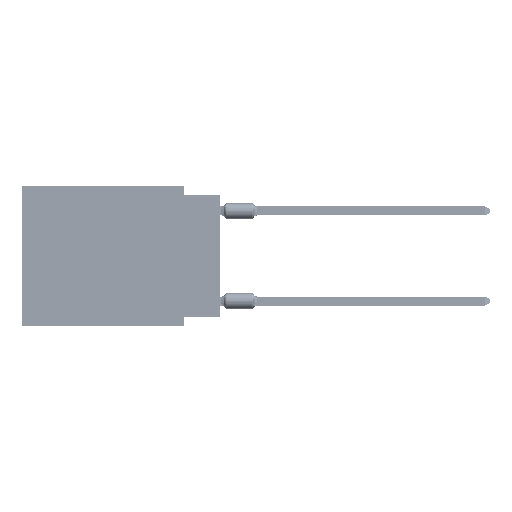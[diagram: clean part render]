
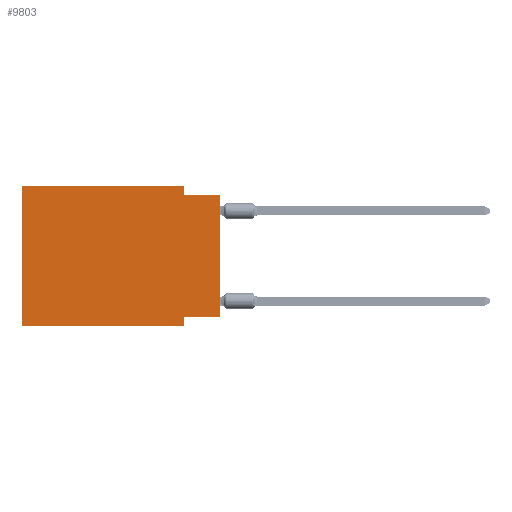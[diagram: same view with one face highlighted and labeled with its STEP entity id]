
A CAD part, left-side view. The second image highlights one B-rep face of the part: STEP entity #9803.
In plain terms, the highlighted planar face has unit normal (-1, 0, 0).
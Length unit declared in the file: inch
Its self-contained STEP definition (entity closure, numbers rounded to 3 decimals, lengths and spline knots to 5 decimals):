
#2476 = CARTESIAN_POINT ( 'NONE',  ( 0., 0.55, 0. ) ) ;
#2557 = ORIENTED_EDGE ( 'NONE', *, *, #18526, .F. ) ;
#5214 = VECTOR ( 'NONE', #5764, 39.37008 ) ;
#5764 = DIRECTION ( 'NONE',  ( 0., 0., 1. ) ) ;
#6551 = EDGE_CURVE ( 'NONE', #72906, #56817, #44185, .T. ) ;
#7378 = AXIS2_PLACEMENT_3D ( 'NONE', #44216, #70729, #11184 ) ;
#8874 = DIRECTION ( 'NONE',  ( 0., 1., 0. ) ) ;
#9182 = VERTEX_POINT ( 'NONE', #49129 ) ;
#9803 = ADVANCED_FACE ( 'NONE', ( #65923 ), #12458, .F. ) ;
#10579 = VECTOR ( 'NONE', #21140, 39.37008 ) ;
#11184 = DIRECTION ( 'NONE',  ( 0., 0., -1. ) ) ;
#11274 = DIRECTION ( 'NONE',  ( 0., 0., -1. ) ) ;
#12458 = PLANE ( 'NONE',  #7378 ) ;
#12565 = ORIENTED_EDGE ( 'NONE', *, *, #36062, .F. ) ;
#16744 = LINE ( 'NONE', #42427, #64588 ) ;
#16815 = CARTESIAN_POINT ( 'NONE',  ( 0., 0.55, -0.39 ) ) ;
#18526 = EDGE_CURVE ( 'NONE', #60700, #67785, #37793, .T. ) ;
#18814 = CARTESIAN_POINT ( 'NONE',  ( 0., 0., 0. ) ) ;
#21140 = DIRECTION ( 'NONE',  ( 0., -1., 0. ) ) ;
#21611 = DIRECTION ( 'NONE',  ( 0., 0., 1. ) ) ;
#21660 = EDGE_CURVE ( 'NONE', #38051, #60700, #54175, .T. ) ;
#21987 = CARTESIAN_POINT ( 'NONE',  ( 0., 0., -0.025 ) ) ;
#22419 = DIRECTION ( 'NONE',  ( 0., 0., -1. ) ) ;
#23654 = VERTEX_POINT ( 'NONE', #81023 ) ;
#24294 = VECTOR ( 'NONE', #11274, 39.37008 ) ;
#35028 = ORIENTED_EDGE ( 'NONE', *, *, #42884, .F. ) ;
#35190 = VECTOR ( 'NONE', #60655, 39.37008 ) ;
#36062 = EDGE_CURVE ( 'NONE', #67785, #23654, #40664, .T. ) ;
#36377 = DIRECTION ( 'NONE',  ( 0., -1., 0. ) ) ;
#36753 = VECTOR ( 'NONE', #36377, 39.37008 ) ;
#37793 = LINE ( 'NONE', #82538, #24294 ) ;
#38051 = VERTEX_POINT ( 'NONE', #59621 ) ;
#40232 = CARTESIAN_POINT ( 'NONE',  ( 0., 0.1, -0.39 ) ) ;
#40664 = LINE ( 'NONE', #21987, #35190 ) ;
#41087 = EDGE_LOOP ( 'NONE', ( #51823, #12565, #2557, #74604, #63601, #71920, #53880, #35028 ) ) ;
#42427 = CARTESIAN_POINT ( 'NONE',  ( 0., 0.1, -0.39 ) ) ;
#42884 = EDGE_CURVE ( 'NONE', #85703, #9182, #54952, .T. ) ;
#43072 = EDGE_CURVE ( 'NONE', #85703, #23654, #64460, .T. ) ;
#44185 = LINE ( 'NONE', #16815, #36753 ) ;
#44216 = CARTESIAN_POINT ( 'NONE',  ( 0., 0.55, 0. ) ) ;
#48211 = CARTESIAN_POINT ( 'NONE',  ( 0., 0.1, -0.025 ) ) ;
#49129 = CARTESIAN_POINT ( 'NONE',  ( 0., 0.1, -0.365 ) ) ;
#49330 = CARTESIAN_POINT ( 'NONE',  ( 0., 0.55, -0.39 ) ) ;
#49957 = CARTESIAN_POINT ( 'NONE',  ( 0., 0.1, 0. ) ) ;
#51823 = ORIENTED_EDGE ( 'NONE', *, *, #43072, .T. ) ;
#52406 = VECTOR ( 'NONE', #8874, 39.37008 ) ;
#53577 = EDGE_CURVE ( 'NONE', #9182, #56817, #16744, .T. ) ;
#53880 = ORIENTED_EDGE ( 'NONE', *, *, #53577, .F. ) ;
#54175 = LINE ( 'NONE', #75010, #10579 ) ;
#54952 = LINE ( 'NONE', #81416, #52406 ) ;
#56530 = CARTESIAN_POINT ( 'NONE',  ( 0., 0., -0.365 ) ) ;
#56817 = VERTEX_POINT ( 'NONE', #40232 ) ;
#59621 = CARTESIAN_POINT ( 'NONE',  ( 0., 0.55, 0. ) ) ;
#60655 = DIRECTION ( 'NONE',  ( 0., -1., 0. ) ) ;
#60700 = VERTEX_POINT ( 'NONE', #49957 ) ;
#62084 = EDGE_CURVE ( 'NONE', #72906, #38051, #81098, .T. ) ;
#63601 = ORIENTED_EDGE ( 'NONE', *, *, #62084, .F. ) ;
#64460 = LINE ( 'NONE', #18814, #5214 ) ;
#64588 = VECTOR ( 'NONE', #22419, 39.37008 ) ;
#65923 = FACE_OUTER_BOUND ( 'NONE', #41087, .T. ) ;
#67785 = VERTEX_POINT ( 'NONE', #48211 ) ;
#70729 = DIRECTION ( 'NONE',  ( 1., 0., 0. ) ) ;
#71920 = ORIENTED_EDGE ( 'NONE', *, *, #6551, .T. ) ;
#72906 = VERTEX_POINT ( 'NONE', #49330 ) ;
#74604 = ORIENTED_EDGE ( 'NONE', *, *, #21660, .F. ) ;
#75010 = CARTESIAN_POINT ( 'NONE',  ( 0., 0.55, 0. ) ) ;
#81023 = CARTESIAN_POINT ( 'NONE',  ( 0., 0., -0.025 ) ) ;
#81098 = LINE ( 'NONE', #2476, #82827 ) ;
#81416 = CARTESIAN_POINT ( 'NONE',  ( 0., 0., -0.365 ) ) ;
#82538 = CARTESIAN_POINT ( 'NONE',  ( 0., 0.1, 0. ) ) ;
#82827 = VECTOR ( 'NONE', #21611, 39.37008 ) ;
#85703 = VERTEX_POINT ( 'NONE', #56530 ) ;
